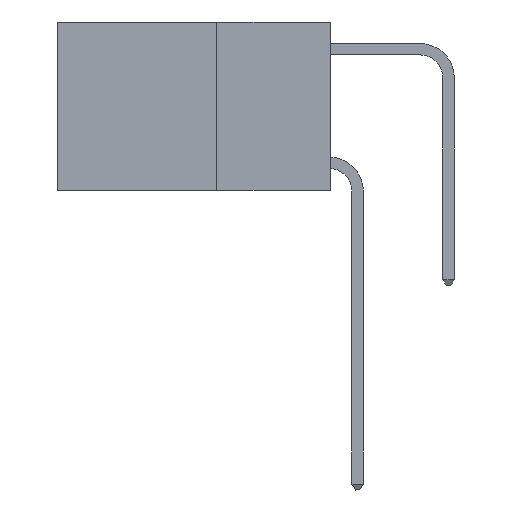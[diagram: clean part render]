
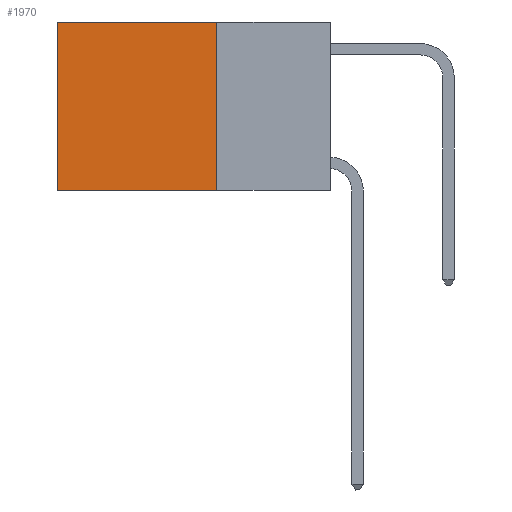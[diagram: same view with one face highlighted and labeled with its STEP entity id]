
A CAD part, left-side view. The second image highlights one B-rep face of the part: STEP entity #1970.
In plain terms, the highlighted planar face has unit normal (-1, 0, 0).
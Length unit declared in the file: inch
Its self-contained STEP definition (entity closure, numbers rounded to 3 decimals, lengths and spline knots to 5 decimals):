
#108 = CARTESIAN_POINT ( 'NONE',  ( 0.2625, 0.6, 0. ) ) ;
#783 = DIRECTION ( 'NONE',  ( 0., 0., -1. ) ) ;
#936 = VERTEX_POINT ( 'NONE', #9863 ) ;
#959 = ORIENTED_EDGE ( 'NONE', *, *, #15992, .F. ) ;
#1023 = DIRECTION ( 'NONE',  ( 0., 1., 0. ) ) ;
#1083 = PLANE ( 'NONE',  #7947 ) ;
#1970 = ADVANCED_FACE ( 'NONE', ( #8889 ), #1083, .F. ) ;
#2271 = VERTEX_POINT ( 'NONE', #11650 ) ;
#2310 = DIRECTION ( 'NONE',  ( 0., 0., -1. ) ) ;
#2671 = CARTESIAN_POINT ( 'NONE',  ( 0.2625, 0.25, -0.37 ) ) ;
#3799 = EDGE_CURVE ( 'NONE', #936, #16307, #3948, .T. ) ;
#3948 = LINE ( 'NONE', #13511, #4350 ) ;
#4350 = VECTOR ( 'NONE', #2310, 39.37008 ) ;
#4678 = CARTESIAN_POINT ( 'NONE',  ( 0.2625, 0.6, 0. ) ) ;
#5028 = EDGE_CURVE ( 'NONE', #20091, #2271, #9206, .T. ) ;
#6060 = LINE ( 'NONE', #18745, #19240 ) ;
#7337 = CARTESIAN_POINT ( 'NONE',  ( 0.2625, 0.25, 0. ) ) ;
#7483 = LINE ( 'NONE', #10681, #12919 ) ;
#7947 = AXIS2_PLACEMENT_3D ( 'NONE', #7337, #13642, #783 ) ;
#8353 = ORIENTED_EDGE ( 'NONE', *, *, #5028, .T. ) ;
#8889 = FACE_OUTER_BOUND ( 'NONE', #19123, .T. ) ;
#9206 = LINE ( 'NONE', #4678, #19838 ) ;
#9863 = CARTESIAN_POINT ( 'NONE',  ( 0.2625, 0.25, 0. ) ) ;
#10681 = CARTESIAN_POINT ( 'NONE',  ( 0.2625, 0.25, 0. ) ) ;
#11586 = EDGE_CURVE ( 'NONE', #936, #20091, #7483, .T. ) ;
#11650 = CARTESIAN_POINT ( 'NONE',  ( 0.2625, 0.6, -0.37 ) ) ;
#12919 = VECTOR ( 'NONE', #1023, 39.37008 ) ;
#13462 = ORIENTED_EDGE ( 'NONE', *, *, #11586, .T. ) ;
#13511 = CARTESIAN_POINT ( 'NONE',  ( 0.2625, 0.25, 0. ) ) ;
#13642 = DIRECTION ( 'NONE',  ( 1., 0., 0. ) ) ;
#15545 = DIRECTION ( 'NONE',  ( 0., 1., 0. ) ) ;
#15992 = EDGE_CURVE ( 'NONE', #16307, #2271, #6060, .T. ) ;
#16307 = VERTEX_POINT ( 'NONE', #2671 ) ;
#16509 = ORIENTED_EDGE ( 'NONE', *, *, #3799, .F. ) ;
#17375 = DIRECTION ( 'NONE',  ( 0., 0., -1. ) ) ;
#18745 = CARTESIAN_POINT ( 'NONE',  ( 0.2625, 0.25, -0.37 ) ) ;
#19123 = EDGE_LOOP ( 'NONE', ( #8353, #959, #16509, #13462 ) ) ;
#19240 = VECTOR ( 'NONE', #15545, 39.37008 ) ;
#19838 = VECTOR ( 'NONE', #17375, 39.37008 ) ;
#20091 = VERTEX_POINT ( 'NONE', #108 ) ;
